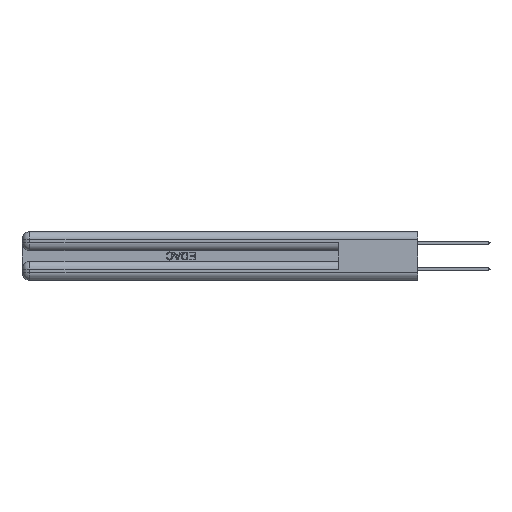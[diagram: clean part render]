
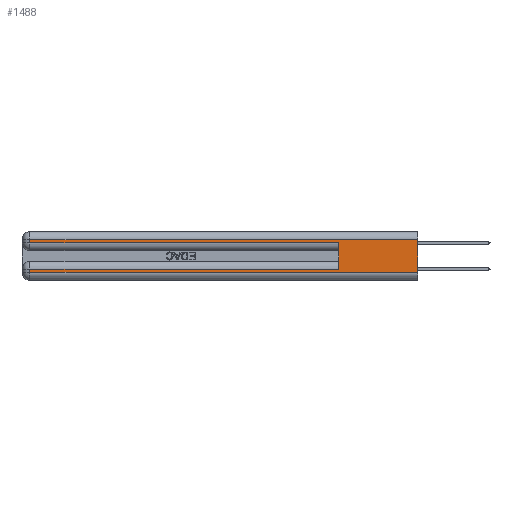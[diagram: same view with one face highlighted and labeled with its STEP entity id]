
A CAD part, left-side view. The second image highlights one B-rep face of the part: STEP entity #1488.
In plain terms, the highlighted planar face has unit normal (-1, 0, 0).
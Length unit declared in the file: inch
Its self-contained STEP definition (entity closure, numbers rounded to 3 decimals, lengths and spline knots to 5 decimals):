
#137 = VECTOR ( 'NONE', #26431, 39.37008 ) ;
#341 = ORIENTED_EDGE ( 'NONE', *, *, #46160, .T. ) ;
#925 = CARTESIAN_POINT ( 'NONE',  ( 0., 2.94, 0.085 ) ) ;
#1105 = CARTESIAN_POINT ( 'NONE',  ( 0., 0., 0.06 ) ) ;
#1438 = DIRECTION ( 'NONE',  ( 0., -1., 0. ) ) ;
#1488 = ADVANCED_FACE ( 'NONE', ( #16456 ), #36189, .F. ) ;
#2569 = LINE ( 'NONE', #49707, #137 ) ;
#2852 = EDGE_CURVE ( 'NONE', #35458, #26816, #9572, .T. ) ;
#3186 = CARTESIAN_POINT ( 'NONE',  ( 0., 0.6, 0.145 ) ) ;
#3508 = CARTESIAN_POINT ( 'NONE',  ( 0., 0., 0.06 ) ) ;
#3846 = EDGE_CURVE ( 'NONE', #14490, #26816, #26159, .T. ) ;
#4102 = VECTOR ( 'NONE', #34501, 39.37008 ) ;
#6297 = ORIENTED_EDGE ( 'NONE', *, *, #46220, .T. ) ;
#7083 = DIRECTION ( 'NONE',  ( 0., 0., -1. ) ) ;
#7443 = VECTOR ( 'NONE', #27935, 39.37008 ) ;
#8119 = EDGE_CURVE ( 'NONE', #34148, #16726, #18351, .T. ) ;
#8147 = EDGE_LOOP ( 'NONE', ( #42403, #25728, #6297, #46750, #21591, #341, #40784, #21975 ) ) ;
#9572 = LINE ( 'NONE', #1105, #48629 ) ;
#11092 = CARTESIAN_POINT ( 'NONE',  ( 0., 0., 0.37 ) ) ;
#12088 = DIRECTION ( 'NONE',  ( 0., 0., -1. ) ) ;
#12723 = VECTOR ( 'NONE', #12088, 39.37008 ) ;
#14490 = VERTEX_POINT ( 'NONE', #42543 ) ;
#15747 = CARTESIAN_POINT ( 'NONE',  ( 0., 2.94, 0.06 ) ) ;
#16456 = FACE_OUTER_BOUND ( 'NONE', #8147, .T. ) ;
#16726 = VERTEX_POINT ( 'NONE', #44968 ) ;
#18351 = LINE ( 'NONE', #3186, #28750 ) ;
#19740 = VECTOR ( 'NONE', #7083, 39.37008 ) ;
#20662 = DIRECTION ( 'NONE',  ( 1., 0., 0. ) ) ;
#20954 = CARTESIAN_POINT ( 'NONE',  ( 0., 2.94, 0.285 ) ) ;
#21591 = ORIENTED_EDGE ( 'NONE', *, *, #8119, .F. ) ;
#21650 = LINE ( 'NONE', #36627, #32008 ) ;
#21975 = ORIENTED_EDGE ( 'NONE', *, *, #2852, .T. ) ;
#23126 = LINE ( 'NONE', #27652, #12723 ) ;
#24035 = CARTESIAN_POINT ( 'NONE',  ( 0., 0., 0.31 ) ) ;
#25728 = ORIENTED_EDGE ( 'NONE', *, *, #46449, .T. ) ;
#26159 = LINE ( 'NONE', #11092, #4102 ) ;
#26431 = DIRECTION ( 'NONE',  ( 0., 1., 0. ) ) ;
#26816 = VERTEX_POINT ( 'NONE', #3508 ) ;
#27652 = CARTESIAN_POINT ( 'NONE',  ( 0., 2.94, 0.37 ) ) ;
#27935 = DIRECTION ( 'NONE',  ( 0., 1., 0. ) ) ;
#28471 = DIRECTION ( 'NONE',  ( 0., -1., 0. ) ) ;
#28636 = CARTESIAN_POINT ( 'NONE',  ( 0., 0.6, 0.085 ) ) ;
#28750 = VECTOR ( 'NONE', #30540, 39.37008 ) ;
#30540 = DIRECTION ( 'NONE',  ( 0., 0., 1. ) ) ;
#32008 = VECTOR ( 'NONE', #1438, 39.37008 ) ;
#34148 = VERTEX_POINT ( 'NONE', #28636 ) ;
#34160 = VERTEX_POINT ( 'NONE', #20954 ) ;
#34501 = DIRECTION ( 'NONE',  ( 0., 0., -1. ) ) ;
#35458 = VERTEX_POINT ( 'NONE', #15747 ) ;
#36189 = PLANE ( 'NONE',  #48464 ) ;
#36627 = CARTESIAN_POINT ( 'NONE',  ( 0., 0., 0.285 ) ) ;
#36808 = VERTEX_POINT ( 'NONE', #925 ) ;
#38186 = EDGE_CURVE ( 'NONE', #34160, #16726, #21650, .T. ) ;
#38323 = CARTESIAN_POINT ( 'NONE',  ( 0., 2.94, 0.37 ) ) ;
#38602 = LINE ( 'NONE', #24035, #7443 ) ;
#40784 = ORIENTED_EDGE ( 'NONE', *, *, #48543, .T. ) ;
#42403 = ORIENTED_EDGE ( 'NONE', *, *, #3846, .F. ) ;
#42543 = CARTESIAN_POINT ( 'NONE',  ( 0., 0., 0.31 ) ) ;
#43982 = CARTESIAN_POINT ( 'NONE',  ( 0., 0., 0.37 ) ) ;
#44968 = CARTESIAN_POINT ( 'NONE',  ( 0., 0.6, 0.285 ) ) ;
#45080 = VERTEX_POINT ( 'NONE', #49638 ) ;
#46160 = EDGE_CURVE ( 'NONE', #34148, #36808, #2569, .T. ) ;
#46220 = EDGE_CURVE ( 'NONE', #45080, #34160, #49562, .T. ) ;
#46449 = EDGE_CURVE ( 'NONE', #14490, #45080, #38602, .T. ) ;
#46750 = ORIENTED_EDGE ( 'NONE', *, *, #38186, .T. ) ;
#47910 = DIRECTION ( 'NONE',  ( 0., 0., -1. ) ) ;
#48464 = AXIS2_PLACEMENT_3D ( 'NONE', #43982, #20662, #47910 ) ;
#48543 = EDGE_CURVE ( 'NONE', #36808, #35458, #23126, .T. ) ;
#48629 = VECTOR ( 'NONE', #28471, 39.37008 ) ;
#49562 = LINE ( 'NONE', #38323, #19740 ) ;
#49638 = CARTESIAN_POINT ( 'NONE',  ( 0., 2.94, 0.31 ) ) ;
#49707 = CARTESIAN_POINT ( 'NONE',  ( 0., 0., 0.085 ) ) ;
